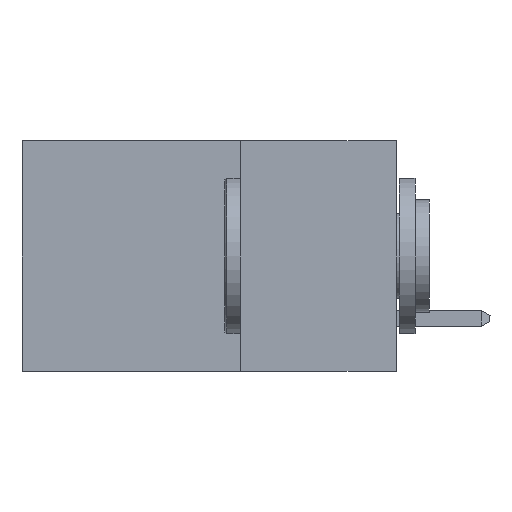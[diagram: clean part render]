
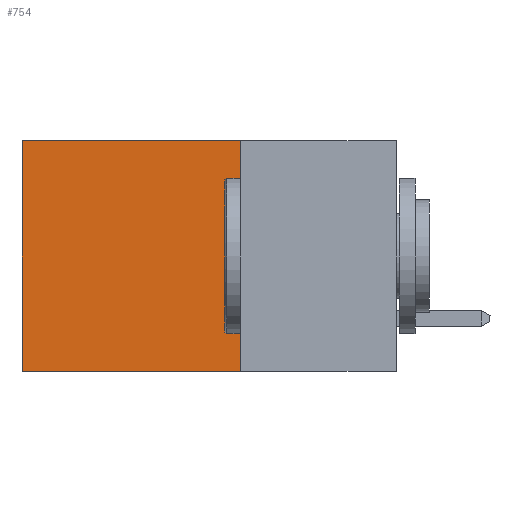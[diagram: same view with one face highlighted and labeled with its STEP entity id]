
A CAD part, left-side view. The second image highlights one B-rep face of the part: STEP entity #754.
In plain terms, the highlighted planar face has unit normal (-1, 0, 0).
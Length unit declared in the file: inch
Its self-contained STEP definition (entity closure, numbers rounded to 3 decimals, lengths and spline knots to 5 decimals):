
#117 = LINE ( 'NONE', #6755, #2436 ) ;
#600 = CARTESIAN_POINT ( 'NONE',  ( 0.2615, 0.6, 0. ) ) ;
#651 = VERTEX_POINT ( 'NONE', #4261 ) ;
#754 = ADVANCED_FACE ( 'NONE', ( #4548 ), #6980, .F. ) ;
#1016 = VECTOR ( 'NONE', #2882, 39.37008 ) ;
#1520 = VERTEX_POINT ( 'NONE', #600 ) ;
#2212 = VERTEX_POINT ( 'NONE', #7317 ) ;
#2436 = VECTOR ( 'NONE', #6883, 39.37008 ) ;
#2882 = DIRECTION ( 'NONE',  ( 0., 1., 0. ) ) ;
#3528 = LINE ( 'NONE', #3760, #1016 ) ;
#3639 = CARTESIAN_POINT ( 'NONE',  ( 0.2615, 0.6, -0.37 ) ) ;
#3643 = EDGE_LOOP ( 'NONE', ( #8993, #8819, #5862, #8534 ) ) ;
#3760 = CARTESIAN_POINT ( 'NONE',  ( 0.2615, 0.25, 0. ) ) ;
#4066 = LINE ( 'NONE', #3639, #6324 ) ;
#4261 = CARTESIAN_POINT ( 'NONE',  ( 0.2615, 0.25, 0. ) ) ;
#4548 = FACE_OUTER_BOUND ( 'NONE', #3643, .T. ) ;
#4579 = DIRECTION ( 'NONE',  ( 0., 0., -1. ) ) ;
#5074 = VERTEX_POINT ( 'NONE', #9656 ) ;
#5205 = AXIS2_PLACEMENT_3D ( 'NONE', #7268, #7244, #7435 ) ;
#5862 = ORIENTED_EDGE ( 'NONE', *, *, #10486, .F. ) ;
#6324 = VECTOR ( 'NONE', #4579, 39.37008 ) ;
#6755 = CARTESIAN_POINT ( 'NONE',  ( 0.2615, 0.25, -0.37 ) ) ;
#6883 = DIRECTION ( 'NONE',  ( 0., 1., 0. ) ) ;
#6980 = PLANE ( 'NONE',  #5205 ) ;
#7244 = DIRECTION ( 'NONE',  ( 1., 0., 0. ) ) ;
#7268 = CARTESIAN_POINT ( 'NONE',  ( 0.2615, 0.25, -0.37 ) ) ;
#7317 = CARTESIAN_POINT ( 'NONE',  ( 0.2615, 0.6, -0.37 ) ) ;
#7353 = EDGE_CURVE ( 'NONE', #5074, #2212, #117, .T. ) ;
#7435 = DIRECTION ( 'NONE',  ( 0., 0., -1. ) ) ;
#7755 = CARTESIAN_POINT ( 'NONE',  ( 0.2615, 0.25, -0.37 ) ) ;
#8534 = ORIENTED_EDGE ( 'NONE', *, *, #9076, .T. ) ;
#8645 = DIRECTION ( 'NONE',  ( 0., 0., -1. ) ) ;
#8768 = VECTOR ( 'NONE', #8645, 39.37008 ) ;
#8819 = ORIENTED_EDGE ( 'NONE', *, *, #7353, .F. ) ;
#8993 = ORIENTED_EDGE ( 'NONE', *, *, #10931, .T. ) ;
#9076 = EDGE_CURVE ( 'NONE', #651, #1520, #3528, .T. ) ;
#9656 = CARTESIAN_POINT ( 'NONE',  ( 0.2615, 0.25, -0.37 ) ) ;
#10486 = EDGE_CURVE ( 'NONE', #651, #5074, #11312, .T. ) ;
#10931 = EDGE_CURVE ( 'NONE', #1520, #2212, #4066, .T. ) ;
#11312 = LINE ( 'NONE', #7755, #8768 ) ;
